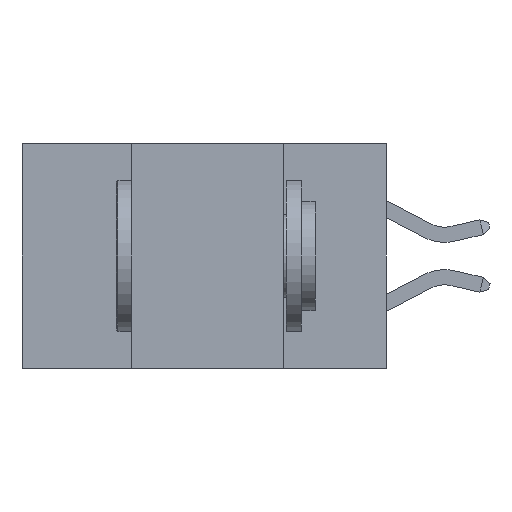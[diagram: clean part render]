
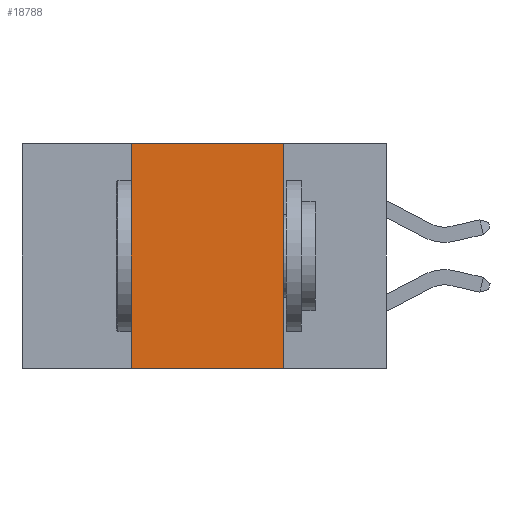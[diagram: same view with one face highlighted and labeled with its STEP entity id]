
A CAD part, left-side view. The second image highlights one B-rep face of the part: STEP entity #18788.
In plain terms, the highlighted planar face has unit normal (-1, 0, 0).
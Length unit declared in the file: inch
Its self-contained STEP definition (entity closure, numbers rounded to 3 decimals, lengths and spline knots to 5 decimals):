
#1567 = VERTEX_POINT ( 'NONE', #10155 ) ;
#1706 = CARTESIAN_POINT ( 'NONE',  ( 0., 0.6, 0. ) ) ;
#2441 = VECTOR ( 'NONE', #7028, 39.37008 ) ;
#2917 = LINE ( 'NONE', #16430, #7603 ) ;
#5254 = LINE ( 'NONE', #21129, #19469 ) ;
#5691 = ORIENTED_EDGE ( 'NONE', *, *, #23929, .F. ) ;
#6013 = CARTESIAN_POINT ( 'NONE',  ( 0., 0.17, -0.37 ) ) ;
#7028 = DIRECTION ( 'NONE',  ( 0., 0., 1. ) ) ;
#7603 = VECTOR ( 'NONE', #23911, 39.37008 ) ;
#7717 = DIRECTION ( 'NONE',  ( 0., -1., 0. ) ) ;
#8232 = PLANE ( 'NONE',  #12178 ) ;
#9959 = CARTESIAN_POINT ( 'NONE',  ( 0., 0.42, -0.37 ) ) ;
#10155 = CARTESIAN_POINT ( 'NONE',  ( 0., 0.42, 0. ) ) ;
#10221 = DIRECTION ( 'NONE',  ( 0., 0., -1. ) ) ;
#10241 = ORIENTED_EDGE ( 'NONE', *, *, #18608, .F. ) ;
#11697 = VERTEX_POINT ( 'NONE', #22348 ) ;
#12033 = VERTEX_POINT ( 'NONE', #9959 ) ;
#12178 = AXIS2_PLACEMENT_3D ( 'NONE', #17919, #21685, #10221 ) ;
#13387 = VERTEX_POINT ( 'NONE', #6013 ) ;
#13632 = EDGE_CURVE ( 'NONE', #11697, #13387, #2917, .T. ) ;
#15005 = VECTOR ( 'NONE', #7717, 39.37008 ) ;
#15891 = FACE_OUTER_BOUND ( 'NONE', #22628, .T. ) ;
#16430 = CARTESIAN_POINT ( 'NONE',  ( 0., 0.17, -0.37 ) ) ;
#16661 = CARTESIAN_POINT ( 'NONE',  ( 0., 0.42, -0.37 ) ) ;
#17214 = ORIENTED_EDGE ( 'NONE', *, *, #24081, .T. ) ;
#17919 = CARTESIAN_POINT ( 'NONE',  ( 0., 0.6, 0. ) ) ;
#18608 = EDGE_CURVE ( 'NONE', #1567, #11697, #20072, .T. ) ;
#18788 = ADVANCED_FACE ( 'NONE', ( #15891 ), #8232, .F. ) ;
#19237 = DIRECTION ( 'NONE',  ( 0., -1., 0. ) ) ;
#19284 = ORIENTED_EDGE ( 'NONE', *, *, #13632, .F. ) ;
#19469 = VECTOR ( 'NONE', #19237, 39.37008 ) ;
#20072 = LINE ( 'NONE', #1706, #15005 ) ;
#21129 = CARTESIAN_POINT ( 'NONE',  ( 0., 0.6, -0.37 ) ) ;
#21685 = DIRECTION ( 'NONE',  ( 1., 0., 0. ) ) ;
#22348 = CARTESIAN_POINT ( 'NONE',  ( 0., 0.17, 0. ) ) ;
#22628 = EDGE_LOOP ( 'NONE', ( #19284, #10241, #5691, #17214 ) ) ;
#22967 = LINE ( 'NONE', #16661, #2441 ) ;
#23911 = DIRECTION ( 'NONE',  ( 0., 0., -1. ) ) ;
#23929 = EDGE_CURVE ( 'NONE', #12033, #1567, #22967, .T. ) ;
#24081 = EDGE_CURVE ( 'NONE', #12033, #13387, #5254, .T. ) ;
